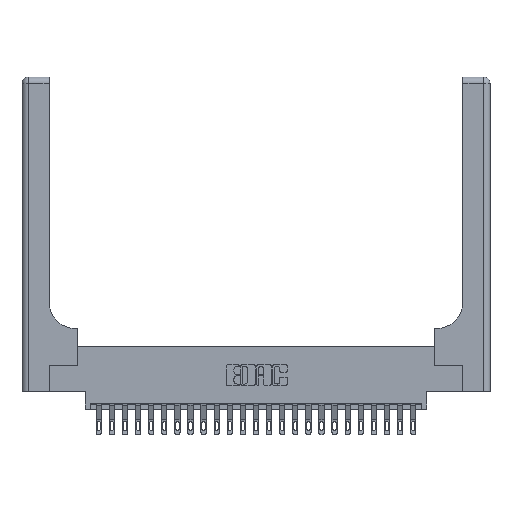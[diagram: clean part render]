
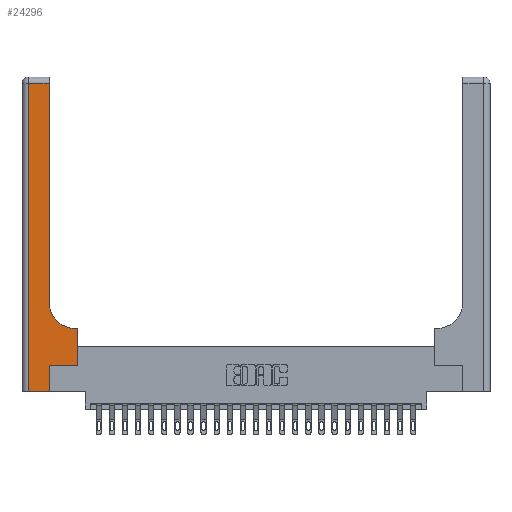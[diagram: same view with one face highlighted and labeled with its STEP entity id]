
A CAD part, top view. The second image highlights one B-rep face of the part: STEP entity #24296.
In plain terms, the highlighted planar face has unit normal (0, 0, 1).
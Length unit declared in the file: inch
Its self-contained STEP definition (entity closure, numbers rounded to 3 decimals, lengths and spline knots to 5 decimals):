
#133 = EDGE_CURVE ( 'NONE', #14245, #15480, #8097, .T. ) ;
#164 = CARTESIAN_POINT ( 'NONE',  ( 0.265, 0., 0.37 ) ) ;
#580 = CARTESIAN_POINT ( 'NONE',  ( 0.06, 2.94, 0.37 ) ) ;
#1755 = VECTOR ( 'NONE', #7642, 39.37008 ) ;
#2571 = DIRECTION ( 'NONE',  ( -1., 0., 0. ) ) ;
#2811 = CARTESIAN_POINT ( 'NONE',  ( 0.51, 0.6, 0.37 ) ) ;
#3188 = CARTESIAN_POINT ( 'NONE',  ( 0., 0., 0.37 ) ) ;
#3480 = VECTOR ( 'NONE', #17622, 39.37008 ) ;
#3849 = EDGE_CURVE ( 'NONE', #21425, #18685, #17387, .T. ) ;
#4236 = VECTOR ( 'NONE', #14149, 39.37008 ) ;
#4375 = CARTESIAN_POINT ( 'NONE',  ( 0.528, 0.25, 0.37 ) ) ;
#4425 = VERTEX_POINT ( 'NONE', #5737 ) ;
#4836 = ORIENTED_EDGE ( 'NONE', *, *, #18745, .T. ) ;
#5241 = CARTESIAN_POINT ( 'NONE',  ( 0.26, 0.85, 0.37 ) ) ;
#5263 = ORIENTED_EDGE ( 'NONE', *, *, #18404, .T. ) ;
#5379 = EDGE_CURVE ( 'NONE', #21136, #7621, #6969, .T. ) ;
#5737 = CARTESIAN_POINT ( 'NONE',  ( 0.265, 0., 0.37 ) ) ;
#5746 = DIRECTION ( 'NONE',  ( 0., 0., -1. ) ) ;
#6288 = CARTESIAN_POINT ( 'NONE',  ( 0.528, 0.6, 0.37 ) ) ;
#6774 = LINE ( 'NONE', #8653, #4236 ) ;
#6969 = CIRCLE ( 'NONE', #20934, 0.25 ) ;
#7087 = DIRECTION ( 'NONE',  ( 0., -1., 0. ) ) ;
#7413 = CARTESIAN_POINT ( 'NONE',  ( 0.265, 0.25, 0.37 ) ) ;
#7473 = LINE ( 'NONE', #24073, #22496 ) ;
#7621 = VERTEX_POINT ( 'NONE', #5241 ) ;
#7642 = DIRECTION ( 'NONE',  ( 0., 1., 0. ) ) ;
#8097 = LINE ( 'NONE', #15719, #18992 ) ;
#8653 = CARTESIAN_POINT ( 'NONE',  ( 0.26, 3., 0.37 ) ) ;
#9396 = LINE ( 'NONE', #164, #1755 ) ;
#9932 = LINE ( 'NONE', #13576, #22806 ) ;
#10145 = DIRECTION ( 'NONE',  ( 1., 0., 0. ) ) ;
#11877 = CARTESIAN_POINT ( 'NONE',  ( 0., 3., 0.37 ) ) ;
#12002 = CARTESIAN_POINT ( 'NONE',  ( 0.51, 0.85, 0.37 ) ) ;
#13576 = CARTESIAN_POINT ( 'NONE',  ( 0.528, 0.25, 0.37 ) ) ;
#13687 = DIRECTION ( 'NONE',  ( 0., 1., 0. ) ) ;
#14149 = DIRECTION ( 'NONE',  ( 0., 1., 0. ) ) ;
#14245 = VERTEX_POINT ( 'NONE', #21574 ) ;
#14501 = VECTOR ( 'NONE', #22892, 39.37008 ) ;
#14766 = ORIENTED_EDGE ( 'NONE', *, *, #20120, .T. ) ;
#15480 = VERTEX_POINT ( 'NONE', #580 ) ;
#15539 = LINE ( 'NONE', #23026, #3480 ) ;
#15719 = CARTESIAN_POINT ( 'NONE',  ( 0., 2.94, 0.37 ) ) ;
#15729 = EDGE_CURVE ( 'NONE', #19973, #4425, #20431, .T. ) ;
#16701 = DIRECTION ( 'NONE',  ( 1., 0., 0. ) ) ;
#17051 = EDGE_CURVE ( 'NONE', #15480, #19973, #7473, .T. ) ;
#17387 = LINE ( 'NONE', #7413, #14501 ) ;
#17596 = PLANE ( 'NONE',  #22872 ) ;
#17622 = DIRECTION ( 'NONE',  ( -1., 0., 0. ) ) ;
#18024 = VECTOR ( 'NONE', #16701, 39.37008 ) ;
#18256 = ORIENTED_EDGE ( 'NONE', *, *, #21711, .T. ) ;
#18404 = EDGE_CURVE ( 'NONE', #18685, #19932, #9932, .T. ) ;
#18685 = VERTEX_POINT ( 'NONE', #4375 ) ;
#18745 = EDGE_CURVE ( 'NONE', #19932, #21136, #15539, .T. ) ;
#18825 = ORIENTED_EDGE ( 'NONE', *, *, #15729, .T. ) ;
#18992 = VECTOR ( 'NONE', #2571, 39.37008 ) ;
#19529 = CARTESIAN_POINT ( 'NONE',  ( 0.06, 0., 0.37 ) ) ;
#19629 = DIRECTION ( 'NONE',  ( 0., 0., -1. ) ) ;
#19856 = ORIENTED_EDGE ( 'NONE', *, *, #17051, .T. ) ;
#19932 = VERTEX_POINT ( 'NONE', #6288 ) ;
#19973 = VERTEX_POINT ( 'NONE', #19529 ) ;
#20120 = EDGE_CURVE ( 'NONE', #7621, #14245, #6774, .T. ) ;
#20431 = LINE ( 'NONE', #3188, #18024 ) ;
#20835 = ORIENTED_EDGE ( 'NONE', *, *, #5379, .T. ) ;
#20867 = FACE_OUTER_BOUND ( 'NONE', #24232, .T. ) ;
#20934 = AXIS2_PLACEMENT_3D ( 'NONE', #12002, #19629, #10145 ) ;
#21008 = DIRECTION ( 'NONE',  ( -1., 0., 0. ) ) ;
#21136 = VERTEX_POINT ( 'NONE', #2811 ) ;
#21425 = VERTEX_POINT ( 'NONE', #21523 ) ;
#21523 = CARTESIAN_POINT ( 'NONE',  ( 0.265, 0.25, 0.37 ) ) ;
#21574 = CARTESIAN_POINT ( 'NONE',  ( 0.26, 2.94, 0.37 ) ) ;
#21601 = ORIENTED_EDGE ( 'NONE', *, *, #3849, .T. ) ;
#21711 = EDGE_CURVE ( 'NONE', #4425, #21425, #9396, .T. ) ;
#22011 = ORIENTED_EDGE ( 'NONE', *, *, #133, .T. ) ;
#22496 = VECTOR ( 'NONE', #7087, 39.37008 ) ;
#22806 = VECTOR ( 'NONE', #13687, 39.37008 ) ;
#22872 = AXIS2_PLACEMENT_3D ( 'NONE', #11877, #5746, #21008 ) ;
#22892 = DIRECTION ( 'NONE',  ( 1., 0., 0. ) ) ;
#23026 = CARTESIAN_POINT ( 'NONE',  ( 0.26, 0.6, 0.37 ) ) ;
#24073 = CARTESIAN_POINT ( 'NONE',  ( 0.06, 3., 0.37 ) ) ;
#24232 = EDGE_LOOP ( 'NONE', ( #14766, #22011, #19856, #18825, #18256, #21601, #5263, #4836, #20835 ) ) ;
#24296 = ADVANCED_FACE ( 'NONE', ( #20867 ), #17596, .F. ) ;
